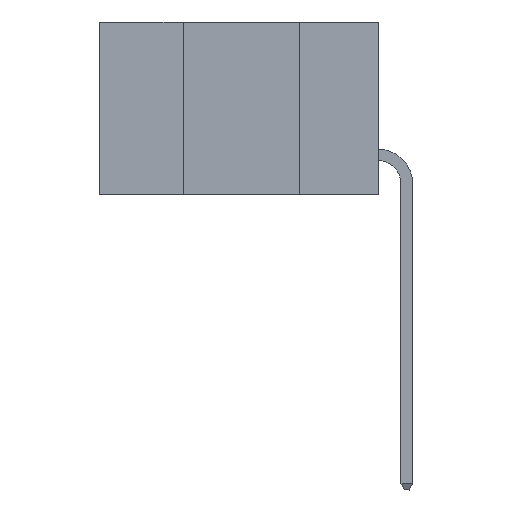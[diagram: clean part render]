
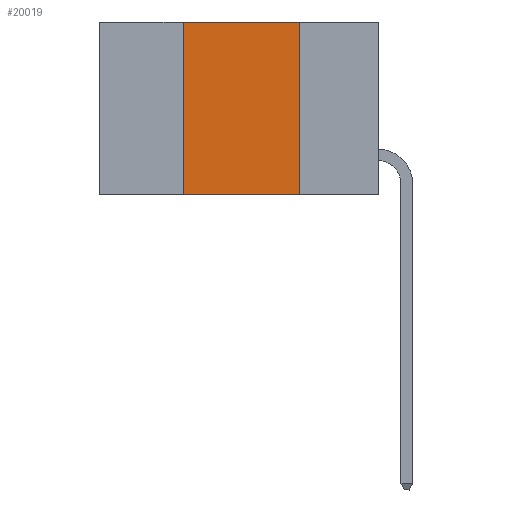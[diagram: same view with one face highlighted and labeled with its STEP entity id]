
A CAD part, left-side view. The second image highlights one B-rep face of the part: STEP entity #20019.
In plain terms, the highlighted planar face has unit normal (-1, 0, 0).
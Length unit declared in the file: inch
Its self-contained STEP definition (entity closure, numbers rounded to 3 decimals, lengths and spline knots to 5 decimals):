
#313 = VECTOR ( 'NONE', #16008, 39.37008 ) ;
#547 = CARTESIAN_POINT ( 'NONE',  ( 0., 0.42, -0.37 ) ) ;
#627 = DIRECTION ( 'NONE',  ( 0., -1., 0. ) ) ;
#1381 = ORIENTED_EDGE ( 'NONE', *, *, #10732, .F. ) ;
#1977 = EDGE_CURVE ( 'NONE', #3493, #9079, #9076, .T. ) ;
#2047 = EDGE_CURVE ( 'NONE', #5740, #4505, #7005, .T. ) ;
#2160 = CARTESIAN_POINT ( 'NONE',  ( 0., 0.6, 0. ) ) ;
#3493 = VERTEX_POINT ( 'NONE', #547 ) ;
#3873 = DIRECTION ( 'NONE',  ( 0., 0., 1. ) ) ;
#3944 = VECTOR ( 'NONE', #3873, 39.37008 ) ;
#4505 = VERTEX_POINT ( 'NONE', #15671 ) ;
#4731 = PLANE ( 'NONE',  #9758 ) ;
#5422 = ORIENTED_EDGE ( 'NONE', *, *, #1977, .T. ) ;
#5740 = VERTEX_POINT ( 'NONE', #6593 ) ;
#6593 = CARTESIAN_POINT ( 'NONE',  ( 0., 0.42, 0. ) ) ;
#7005 = LINE ( 'NONE', #2160, #20140 ) ;
#8305 = ORIENTED_EDGE ( 'NONE', *, *, #2047, .F. ) ;
#9076 = LINE ( 'NONE', #19917, #16503 ) ;
#9079 = VERTEX_POINT ( 'NONE', #16903 ) ;
#9178 = CARTESIAN_POINT ( 'NONE',  ( 0., 0.17, -0.37 ) ) ;
#9758 = AXIS2_PLACEMENT_3D ( 'NONE', #17026, #11265, #20591 ) ;
#10085 = FACE_OUTER_BOUND ( 'NONE', #10657, .T. ) ;
#10657 = EDGE_LOOP ( 'NONE', ( #20271, #8305, #1381, #5422 ) ) ;
#10732 = EDGE_CURVE ( 'NONE', #3493, #5740, #12564, .T. ) ;
#10786 = LINE ( 'NONE', #9178, #313 ) ;
#11265 = DIRECTION ( 'NONE',  ( 1., 0., 0. ) ) ;
#12564 = LINE ( 'NONE', #19522, #3944 ) ;
#14627 = EDGE_CURVE ( 'NONE', #4505, #9079, #10786, .T. ) ;
#15671 = CARTESIAN_POINT ( 'NONE',  ( 0., 0.17, 0. ) ) ;
#16008 = DIRECTION ( 'NONE',  ( 0., 0., -1. ) ) ;
#16503 = VECTOR ( 'NONE', #627, 39.37008 ) ;
#16903 = CARTESIAN_POINT ( 'NONE',  ( 0., 0.17, -0.37 ) ) ;
#17026 = CARTESIAN_POINT ( 'NONE',  ( 0., 0.6, 0. ) ) ;
#17481 = DIRECTION ( 'NONE',  ( 0., -1., 0. ) ) ;
#19522 = CARTESIAN_POINT ( 'NONE',  ( 0., 0.42, -0.37 ) ) ;
#19917 = CARTESIAN_POINT ( 'NONE',  ( 0., 0.6, -0.37 ) ) ;
#20019 = ADVANCED_FACE ( 'NONE', ( #10085 ), #4731, .F. ) ;
#20140 = VECTOR ( 'NONE', #17481, 39.37008 ) ;
#20271 = ORIENTED_EDGE ( 'NONE', *, *, #14627, .F. ) ;
#20591 = DIRECTION ( 'NONE',  ( 0., 0., -1. ) ) ;
